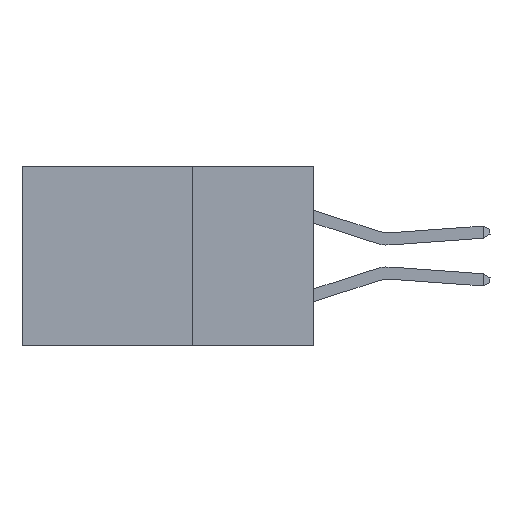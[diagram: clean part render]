
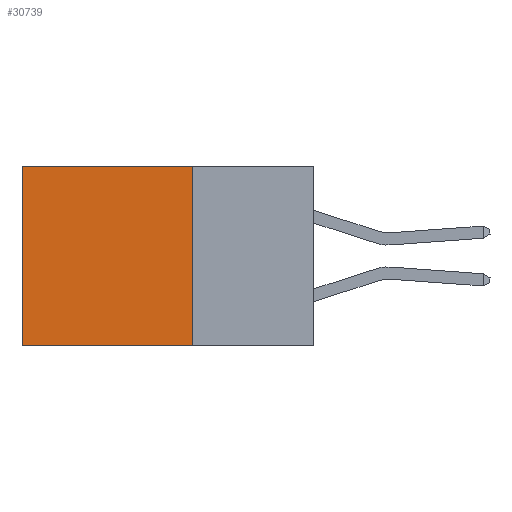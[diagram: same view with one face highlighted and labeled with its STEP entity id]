
A CAD part, left-side view. The second image highlights one B-rep face of the part: STEP entity #30739.
In plain terms, the highlighted planar face has unit normal (-1, 0, 0).
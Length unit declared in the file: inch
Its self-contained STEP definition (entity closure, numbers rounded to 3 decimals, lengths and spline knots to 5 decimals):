
#2145 = VERTEX_POINT ( 'NONE', #31922 ) ;
#4251 = VERTEX_POINT ( 'NONE', #14912 ) ;
#5703 = DIRECTION ( 'NONE',  ( 0., 0., -1. ) ) ;
#6416 = AXIS2_PLACEMENT_3D ( 'NONE', #26524, #12514, #36962 ) ;
#9595 = DIRECTION ( 'NONE',  ( 0., 1., 0. ) ) ;
#10111 = VECTOR ( 'NONE', #11434, 39.37008 ) ;
#10906 = EDGE_CURVE ( 'NONE', #19347, #4251, #42291, .T. ) ;
#11434 = DIRECTION ( 'NONE',  ( 0., 0., -1. ) ) ;
#12514 = DIRECTION ( 'NONE',  ( 1., 0., 0. ) ) ;
#12807 = EDGE_CURVE ( 'NONE', #4251, #27838, #26675, .T. ) ;
#14008 = ORIENTED_EDGE ( 'NONE', *, *, #32100, .F. ) ;
#14912 = CARTESIAN_POINT ( 'NONE',  ( 0.2875, 0.6, 0. ) ) ;
#16442 = ORIENTED_EDGE ( 'NONE', *, *, #10906, .T. ) ;
#17283 = ORIENTED_EDGE ( 'NONE', *, *, #12807, .T. ) ;
#19347 = VERTEX_POINT ( 'NONE', #29041 ) ;
#23942 = VECTOR ( 'NONE', #33787, 39.37008 ) ;
#25400 = EDGE_LOOP ( 'NONE', ( #17283, #14008, #27033, #16442 ) ) ;
#26524 = CARTESIAN_POINT ( 'NONE',  ( 0.2875, 0.25, 0. ) ) ;
#26675 = LINE ( 'NONE', #35923, #10111 ) ;
#26948 = CARTESIAN_POINT ( 'NONE',  ( 0.2875, 0.25, 0. ) ) ;
#27033 = ORIENTED_EDGE ( 'NONE', *, *, #35676, .F. ) ;
#27838 = VERTEX_POINT ( 'NONE', #28274 ) ;
#28274 = CARTESIAN_POINT ( 'NONE',  ( 0.2875, 0.6, -0.37 ) ) ;
#29041 = CARTESIAN_POINT ( 'NONE',  ( 0.2875, 0.25, 0. ) ) ;
#30739 = ADVANCED_FACE ( 'NONE', ( #36623 ), #43659, .F. ) ;
#31922 = CARTESIAN_POINT ( 'NONE',  ( 0.2875, 0.25, -0.37 ) ) ;
#32100 = EDGE_CURVE ( 'NONE', #2145, #27838, #42368, .T. ) ;
#33254 = VECTOR ( 'NONE', #9595, 39.37008 ) ;
#33787 = DIRECTION ( 'NONE',  ( 0., 1., 0. ) ) ;
#35676 = EDGE_CURVE ( 'NONE', #19347, #2145, #41341, .T. ) ;
#35923 = CARTESIAN_POINT ( 'NONE',  ( 0.2875, 0.6, 0. ) ) ;
#36623 = FACE_OUTER_BOUND ( 'NONE', #25400, .T. ) ;
#36962 = DIRECTION ( 'NONE',  ( 0., 0., -1. ) ) ;
#37104 = CARTESIAN_POINT ( 'NONE',  ( 0.2875, 0.25, 0. ) ) ;
#40285 = VECTOR ( 'NONE', #5703, 39.37008 ) ;
#40903 = CARTESIAN_POINT ( 'NONE',  ( 0.2875, 0.25, -0.37 ) ) ;
#41341 = LINE ( 'NONE', #26948, #40285 ) ;
#42291 = LINE ( 'NONE', #37104, #23942 ) ;
#42368 = LINE ( 'NONE', #40903, #33254 ) ;
#43659 = PLANE ( 'NONE',  #6416 ) ;
